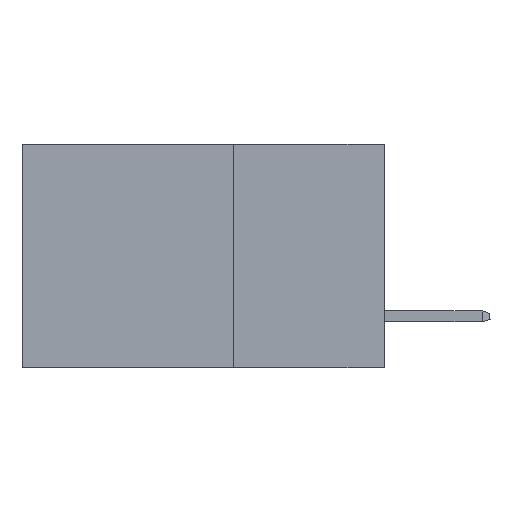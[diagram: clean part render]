
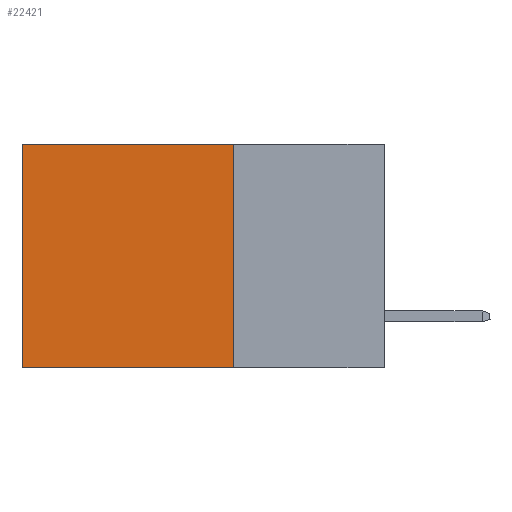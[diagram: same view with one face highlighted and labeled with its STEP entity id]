
A CAD part, left-side view. The second image highlights one B-rep face of the part: STEP entity #22421.
In plain terms, the highlighted planar face has unit normal (-1, 0, 0).
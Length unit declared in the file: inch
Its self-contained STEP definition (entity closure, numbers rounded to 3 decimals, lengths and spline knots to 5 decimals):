
#163 = EDGE_CURVE ( 'NONE', #14314, #16120, #4505, .T. ) ;
#314 = DIRECTION ( 'NONE',  ( 0., 0., -1. ) ) ;
#2416 = EDGE_CURVE ( 'NONE', #5535, #16120, #4397, .T. ) ;
#2555 = DIRECTION ( 'NONE',  ( 0., 0., -1. ) ) ;
#3669 = EDGE_CURVE ( 'NONE', #24033, #14314, #19978, .T. ) ;
#4397 = LINE ( 'NONE', #18505, #15274 ) ;
#4505 = LINE ( 'NONE', #21652, #13664 ) ;
#5369 = AXIS2_PLACEMENT_3D ( 'NONE', #8844, #6672, #314 ) ;
#5535 = VERTEX_POINT ( 'NONE', #10864 ) ;
#6124 = ORIENTED_EDGE ( 'NONE', *, *, #26956, .F. ) ;
#6672 = DIRECTION ( 'NONE',  ( 1., 0., 0. ) ) ;
#7188 = ORIENTED_EDGE ( 'NONE', *, *, #3669, .T. ) ;
#8412 = VECTOR ( 'NONE', #23174, 39.37008 ) ;
#8844 = CARTESIAN_POINT ( 'NONE',  ( 0.298, 0.25, 0. ) ) ;
#10584 = LINE ( 'NONE', #21996, #17711 ) ;
#10864 = CARTESIAN_POINT ( 'NONE',  ( 0.298, 0.25, -0.37 ) ) ;
#12552 = ORIENTED_EDGE ( 'NONE', *, *, #163, .T. ) ;
#13144 = PLANE ( 'NONE',  #5369 ) ;
#13664 = VECTOR ( 'NONE', #15379, 39.37008 ) ;
#13919 = EDGE_LOOP ( 'NONE', ( #12552, #14762, #6124, #7188 ) ) ;
#14314 = VERTEX_POINT ( 'NONE', #19594 ) ;
#14762 = ORIENTED_EDGE ( 'NONE', *, *, #2416, .F. ) ;
#15274 = VECTOR ( 'NONE', #20488, 39.37008 ) ;
#15379 = DIRECTION ( 'NONE',  ( 0., 0., -1. ) ) ;
#16120 = VERTEX_POINT ( 'NONE', #20320 ) ;
#16765 = FACE_OUTER_BOUND ( 'NONE', #13919, .T. ) ;
#17711 = VECTOR ( 'NONE', #2555, 39.37008 ) ;
#18505 = CARTESIAN_POINT ( 'NONE',  ( 0.298, 0.25, -0.37 ) ) ;
#18716 = CARTESIAN_POINT ( 'NONE',  ( 0.298, 0.25, 0. ) ) ;
#19594 = CARTESIAN_POINT ( 'NONE',  ( 0.298, 0.6, 0. ) ) ;
#19978 = LINE ( 'NONE', #18716, #8412 ) ;
#20320 = CARTESIAN_POINT ( 'NONE',  ( 0.298, 0.6, -0.37 ) ) ;
#20488 = DIRECTION ( 'NONE',  ( 0., 1., 0. ) ) ;
#20669 = CARTESIAN_POINT ( 'NONE',  ( 0.298, 0.25, 0. ) ) ;
#21652 = CARTESIAN_POINT ( 'NONE',  ( 0.298, 0.6, 0. ) ) ;
#21996 = CARTESIAN_POINT ( 'NONE',  ( 0.298, 0.25, 0. ) ) ;
#22421 = ADVANCED_FACE ( 'NONE', ( #16765 ), #13144, .F. ) ;
#23174 = DIRECTION ( 'NONE',  ( 0., 1., 0. ) ) ;
#24033 = VERTEX_POINT ( 'NONE', #20669 ) ;
#26956 = EDGE_CURVE ( 'NONE', #24033, #5535, #10584, .T. ) ;
